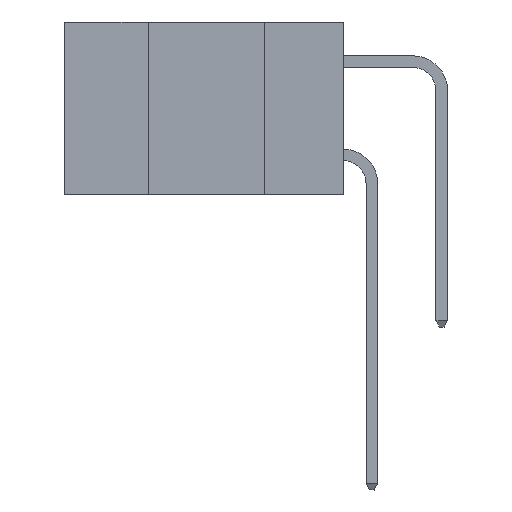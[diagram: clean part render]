
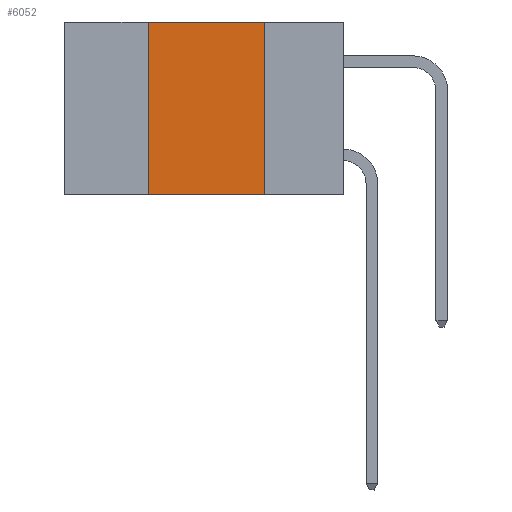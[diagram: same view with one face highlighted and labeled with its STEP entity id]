
A CAD part, left-side view. The second image highlights one B-rep face of the part: STEP entity #6052.
In plain terms, the highlighted planar face has unit normal (-1, 0, 0).
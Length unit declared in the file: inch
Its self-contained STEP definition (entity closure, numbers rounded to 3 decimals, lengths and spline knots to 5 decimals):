
#330 = ORIENTED_EDGE ( 'NONE', *, *, #21956, .T. ) ;
#679 = DIRECTION ( 'NONE',  ( 0., -1., 0. ) ) ;
#1474 = VECTOR ( 'NONE', #21385, 39.37008 ) ;
#1683 = ORIENTED_EDGE ( 'NONE', *, *, #24776, .F. ) ;
#3153 = VERTEX_POINT ( 'NONE', #11894 ) ;
#4103 = LINE ( 'NONE', #10293, #20617 ) ;
#4805 = CARTESIAN_POINT ( 'NONE',  ( 0., 0.6, 0. ) ) ;
#6052 = ADVANCED_FACE ( 'NONE', ( #23238 ), #19326, .F. ) ;
#6473 = VERTEX_POINT ( 'NONE', #22404 ) ;
#8698 = VECTOR ( 'NONE', #679, 39.37008 ) ;
#8888 = AXIS2_PLACEMENT_3D ( 'NONE', #4805, #17303, #18777 ) ;
#10164 = EDGE_CURVE ( 'NONE', #23863, #3153, #4103, .T. ) ;
#10293 = CARTESIAN_POINT ( 'NONE',  ( 0., 0.6, 0. ) ) ;
#10989 = VERTEX_POINT ( 'NONE', #13600 ) ;
#11174 = CARTESIAN_POINT ( 'NONE',  ( 0., 0.6, -0.37 ) ) ;
#11894 = CARTESIAN_POINT ( 'NONE',  ( 0., 0.17, 0. ) ) ;
#13600 = CARTESIAN_POINT ( 'NONE',  ( 0., 0.42, -0.37 ) ) ;
#14421 = ORIENTED_EDGE ( 'NONE', *, *, #22341, .F. ) ;
#14722 = ORIENTED_EDGE ( 'NONE', *, *, #10164, .F. ) ;
#14896 = LINE ( 'NONE', #25516, #16389 ) ;
#15324 = LINE ( 'NONE', #23687, #1474 ) ;
#16389 = VECTOR ( 'NONE', #16783, 39.37008 ) ;
#16783 = DIRECTION ( 'NONE',  ( 0., 0., -1. ) ) ;
#17303 = DIRECTION ( 'NONE',  ( 1., 0., 0. ) ) ;
#17383 = EDGE_LOOP ( 'NONE', ( #14421, #14722, #1683, #330 ) ) ;
#18777 = DIRECTION ( 'NONE',  ( 0., 0., -1. ) ) ;
#19098 = LINE ( 'NONE', #11174, #8698 ) ;
#19326 = PLANE ( 'NONE',  #8888 ) ;
#20617 = VECTOR ( 'NONE', #24562, 39.37008 ) ;
#21385 = DIRECTION ( 'NONE',  ( 0., 0., 1. ) ) ;
#21956 = EDGE_CURVE ( 'NONE', #10989, #6473, #19098, .T. ) ;
#22341 = EDGE_CURVE ( 'NONE', #3153, #6473, #14896, .T. ) ;
#22404 = CARTESIAN_POINT ( 'NONE',  ( 0., 0.17, -0.37 ) ) ;
#23238 = FACE_OUTER_BOUND ( 'NONE', #17383, .T. ) ;
#23687 = CARTESIAN_POINT ( 'NONE',  ( 0., 0.42, -0.37 ) ) ;
#23863 = VERTEX_POINT ( 'NONE', #26447 ) ;
#24562 = DIRECTION ( 'NONE',  ( 0., -1., 0. ) ) ;
#24776 = EDGE_CURVE ( 'NONE', #10989, #23863, #15324, .T. ) ;
#25516 = CARTESIAN_POINT ( 'NONE',  ( 0., 0.17, -0.37 ) ) ;
#26447 = CARTESIAN_POINT ( 'NONE',  ( 0., 0.42, 0. ) ) ;
